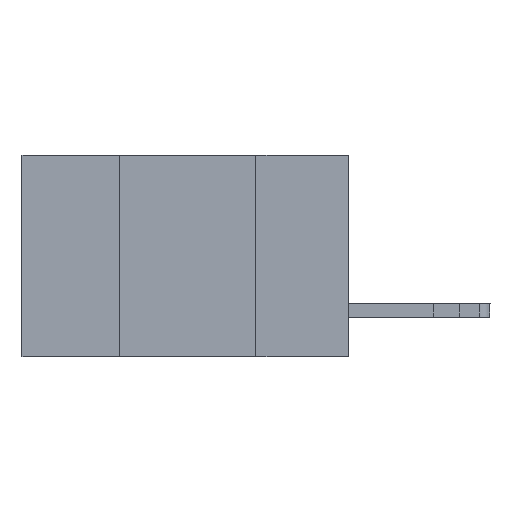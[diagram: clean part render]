
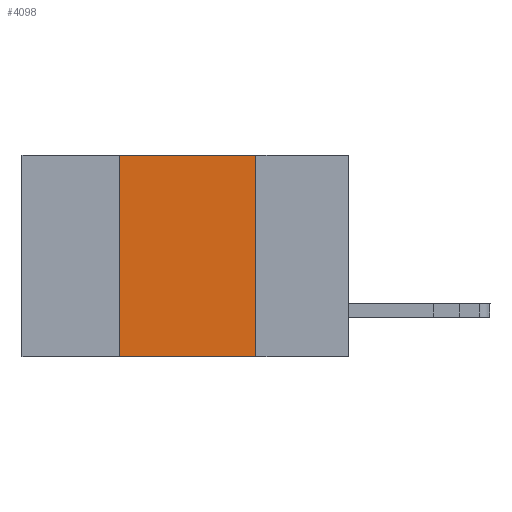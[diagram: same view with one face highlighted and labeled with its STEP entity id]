
A CAD part, left-side view. The second image highlights one B-rep face of the part: STEP entity #4098.
In plain terms, the highlighted planar face has unit normal (-1, 0, 0).
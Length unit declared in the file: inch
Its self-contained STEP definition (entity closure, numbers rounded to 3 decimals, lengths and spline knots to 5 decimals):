
#31 = EDGE_LOOP ( 'NONE', ( #1093, #3802, #11261, #9641 ) ) ;
#233 = CARTESIAN_POINT ( 'NONE',  ( 0., 0.6, 0. ) ) ;
#539 = CARTESIAN_POINT ( 'NONE',  ( 0., 0.42, 0. ) ) ;
#764 = AXIS2_PLACEMENT_3D ( 'NONE', #1657, #1545, #7324 ) ;
#1093 = ORIENTED_EDGE ( 'NONE', *, *, #6198, .F. ) ;
#1545 = DIRECTION ( 'NONE',  ( 1., 0., 0. ) ) ;
#1657 = CARTESIAN_POINT ( 'NONE',  ( 0., 0.6, 0. ) ) ;
#1895 = VERTEX_POINT ( 'NONE', #539 ) ;
#3496 = CARTESIAN_POINT ( 'NONE',  ( 0., 0.6, -0.37 ) ) ;
#3559 = DIRECTION ( 'NONE',  ( 0., -1., 0. ) ) ;
#3602 = FACE_OUTER_BOUND ( 'NONE', #31, .T. ) ;
#3802 = ORIENTED_EDGE ( 'NONE', *, *, #7512, .F. ) ;
#4098 = ADVANCED_FACE ( 'NONE', ( #3602 ), #7360, .F. ) ;
#4433 = VECTOR ( 'NONE', #3559, 39.37008 ) ;
#4749 = LINE ( 'NONE', #3496, #4433 ) ;
#5030 = VERTEX_POINT ( 'NONE', #11779 ) ;
#5312 = VECTOR ( 'NONE', #10089, 39.37008 ) ;
#5847 = EDGE_CURVE ( 'NONE', #5030, #9618, #4749, .T. ) ;
#6106 = VECTOR ( 'NONE', #11200, 39.37008 ) ;
#6198 = EDGE_CURVE ( 'NONE', #10589, #9618, #10356, .T. ) ;
#6264 = EDGE_CURVE ( 'NONE', #5030, #1895, #11220, .T. ) ;
#7324 = DIRECTION ( 'NONE',  ( 0., 0., -1. ) ) ;
#7351 = DIRECTION ( 'NONE',  ( 0., -1., 0. ) ) ;
#7360 = PLANE ( 'NONE',  #764 ) ;
#7512 = EDGE_CURVE ( 'NONE', #1895, #10589, #10554, .T. ) ;
#7824 = CARTESIAN_POINT ( 'NONE',  ( 0., 0.17, 0. ) ) ;
#8046 = VECTOR ( 'NONE', #7351, 39.37008 ) ;
#8161 = CARTESIAN_POINT ( 'NONE',  ( 0., 0.17, -0.37 ) ) ;
#9590 = CARTESIAN_POINT ( 'NONE',  ( 0., 0.42, -0.37 ) ) ;
#9618 = VERTEX_POINT ( 'NONE', #8161 ) ;
#9641 = ORIENTED_EDGE ( 'NONE', *, *, #5847, .T. ) ;
#10089 = DIRECTION ( 'NONE',  ( 0., 0., -1. ) ) ;
#10356 = LINE ( 'NONE', #11354, #5312 ) ;
#10554 = LINE ( 'NONE', #233, #8046 ) ;
#10589 = VERTEX_POINT ( 'NONE', #7824 ) ;
#11200 = DIRECTION ( 'NONE',  ( 0., 0., 1. ) ) ;
#11220 = LINE ( 'NONE', #9590, #6106 ) ;
#11261 = ORIENTED_EDGE ( 'NONE', *, *, #6264, .F. ) ;
#11354 = CARTESIAN_POINT ( 'NONE',  ( 0., 0.17, -0.37 ) ) ;
#11779 = CARTESIAN_POINT ( 'NONE',  ( 0., 0.42, -0.37 ) ) ;
